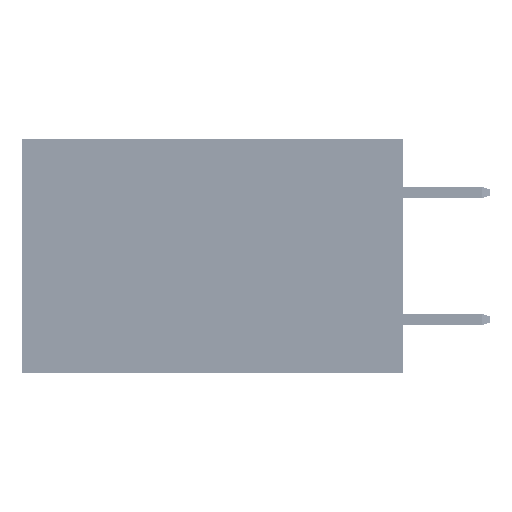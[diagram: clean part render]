
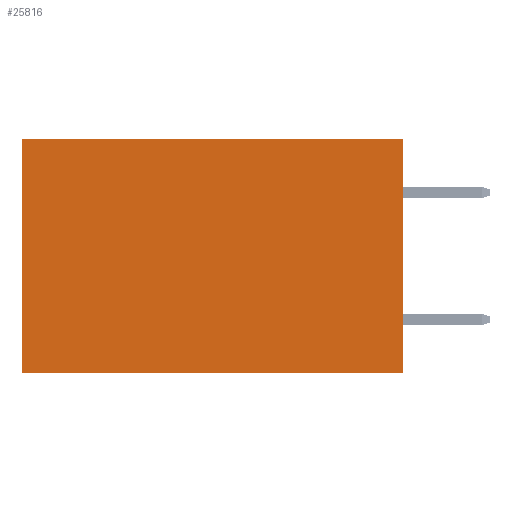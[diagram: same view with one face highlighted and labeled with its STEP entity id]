
A CAD part, left-side view. The second image highlights one B-rep face of the part: STEP entity #25816.
In plain terms, the highlighted planar face has unit normal (-1, 0, 0).
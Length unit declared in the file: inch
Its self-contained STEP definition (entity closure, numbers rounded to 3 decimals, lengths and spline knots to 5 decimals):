
#107 = EDGE_CURVE ( 'NONE', #11364, #18491, #20832, .T. ) ;
#3212 = ORIENTED_EDGE ( 'NONE', *, *, #4403, .F. ) ;
#4403 = EDGE_CURVE ( 'NONE', #33202, #18119, #14902, .T. ) ;
#4690 = EDGE_CURVE ( 'NONE', #18119, #18491, #28612, .T. ) ;
#8295 = LINE ( 'NONE', #12927, #21230 ) ;
#9260 = DIRECTION ( 'NONE',  ( 0., 1., 0. ) ) ;
#9915 = ORIENTED_EDGE ( 'NONE', *, *, #27884, .T. ) ;
#11364 = VERTEX_POINT ( 'NONE', #40819 ) ;
#11473 = CARTESIAN_POINT ( 'NONE',  ( 0.2875, 0., 0. ) ) ;
#12927 = CARTESIAN_POINT ( 'NONE',  ( 0.2875, 0., 0. ) ) ;
#14346 = DIRECTION ( 'NONE',  ( 0., 0., -1. ) ) ;
#14902 = LINE ( 'NONE', #11473, #20968 ) ;
#17075 = ORIENTED_EDGE ( 'NONE', *, *, #4690, .F. ) ;
#18119 = VERTEX_POINT ( 'NONE', #47254 ) ;
#18491 = VERTEX_POINT ( 'NONE', #28247 ) ;
#20104 = EDGE_LOOP ( 'NONE', ( #24764, #17075, #3212, #9915 ) ) ;
#20832 = LINE ( 'NONE', #28722, #42598 ) ;
#20968 = VECTOR ( 'NONE', #29887, 39.37008 ) ;
#21230 = VECTOR ( 'NONE', #9260, 39.37008 ) ;
#24390 = PLANE ( 'NONE',  #29873 ) ;
#24764 = ORIENTED_EDGE ( 'NONE', *, *, #107, .T. ) ;
#25374 = DIRECTION ( 'NONE',  ( 1., 0., 0. ) ) ;
#25816 = ADVANCED_FACE ( 'NONE', ( #27862 ), #24390, .F. ) ;
#27862 = FACE_OUTER_BOUND ( 'NONE', #20104, .T. ) ;
#27884 = EDGE_CURVE ( 'NONE', #33202, #11364, #8295, .T. ) ;
#28247 = CARTESIAN_POINT ( 'NONE',  ( 0.2875, 0.6, -0.37 ) ) ;
#28612 = LINE ( 'NONE', #29104, #36678 ) ;
#28722 = CARTESIAN_POINT ( 'NONE',  ( 0.2875, 0.6, 0. ) ) ;
#29104 = CARTESIAN_POINT ( 'NONE',  ( 0.2875, 0., -0.37 ) ) ;
#29873 = AXIS2_PLACEMENT_3D ( 'NONE', #32012, #25374, #14346 ) ;
#29887 = DIRECTION ( 'NONE',  ( 0., 0., -1. ) ) ;
#32012 = CARTESIAN_POINT ( 'NONE',  ( 0.2875, 0., 0. ) ) ;
#32644 = DIRECTION ( 'NONE',  ( 0., 0., -1. ) ) ;
#33202 = VERTEX_POINT ( 'NONE', #47677 ) ;
#36678 = VECTOR ( 'NONE', #44032, 39.37008 ) ;
#40819 = CARTESIAN_POINT ( 'NONE',  ( 0.2875, 0.6, 0. ) ) ;
#42598 = VECTOR ( 'NONE', #32644, 39.37008 ) ;
#44032 = DIRECTION ( 'NONE',  ( 0., 1., 0. ) ) ;
#47254 = CARTESIAN_POINT ( 'NONE',  ( 0.2875, 0., -0.37 ) ) ;
#47677 = CARTESIAN_POINT ( 'NONE',  ( 0.2875, 0., 0. ) ) ;
